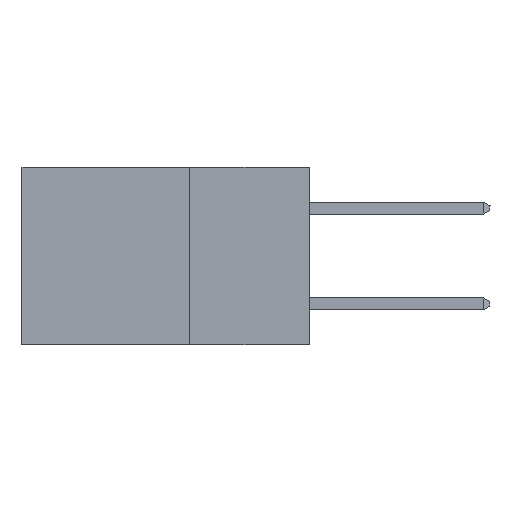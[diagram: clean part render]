
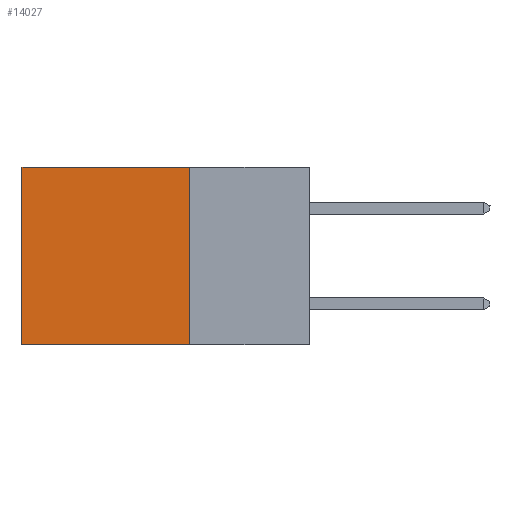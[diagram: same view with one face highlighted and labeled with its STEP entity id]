
A CAD part, left-side view. The second image highlights one B-rep face of the part: STEP entity #14027.
In plain terms, the highlighted planar face has unit normal (-1, 0, 0).
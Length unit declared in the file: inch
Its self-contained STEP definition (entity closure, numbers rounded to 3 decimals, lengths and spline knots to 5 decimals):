
#1872 = DIRECTION ( 'NONE',  ( 0., 1., 0. ) ) ;
#2733 = DIRECTION ( 'NONE',  ( 0., 0., -1. ) ) ;
#2737 = LINE ( 'NONE', #13166, #22405 ) ;
#5017 = AXIS2_PLACEMENT_3D ( 'NONE', #7949, #16722, #25868 ) ;
#5042 = EDGE_CURVE ( 'NONE', #13042, #8518, #17000, .T. ) ;
#5381 = DIRECTION ( 'NONE',  ( 0., 1., 0. ) ) ;
#6493 = EDGE_CURVE ( 'NONE', #26547, #13929, #2737, .T. ) ;
#7454 = PLANE ( 'NONE',  #5017 ) ;
#7816 = EDGE_CURVE ( 'NONE', #26547, #13042, #15989, .T. ) ;
#7836 = DIRECTION ( 'NONE',  ( 0., 0., -1. ) ) ;
#7949 = CARTESIAN_POINT ( 'NONE',  ( 0.2875, 0.25, 0. ) ) ;
#8518 = VERTEX_POINT ( 'NONE', #31159 ) ;
#8764 = ORIENTED_EDGE ( 'NONE', *, *, #28070, .F. ) ;
#11246 = CARTESIAN_POINT ( 'NONE',  ( 0.2875, 0.25, 0. ) ) ;
#12551 = VECTOR ( 'NONE', #5381, 39.37008 ) ;
#13042 = VERTEX_POINT ( 'NONE', #29510 ) ;
#13166 = CARTESIAN_POINT ( 'NONE',  ( 0.2875, 0.25, 0. ) ) ;
#13929 = VERTEX_POINT ( 'NONE', #28037 ) ;
#14027 = ADVANCED_FACE ( 'NONE', ( #21763 ), #7454, .F. ) ;
#15383 = ORIENTED_EDGE ( 'NONE', *, *, #7816, .T. ) ;
#15989 = LINE ( 'NONE', #32851, #12551 ) ;
#16722 = DIRECTION ( 'NONE',  ( 1., 0., 0. ) ) ;
#17000 = LINE ( 'NONE', #24329, #27331 ) ;
#18820 = ORIENTED_EDGE ( 'NONE', *, *, #6493, .F. ) ;
#20356 = EDGE_LOOP ( 'NONE', ( #22489, #8764, #18820, #15383 ) ) ;
#21763 = FACE_OUTER_BOUND ( 'NONE', #20356, .T. ) ;
#22405 = VECTOR ( 'NONE', #7836, 39.37008 ) ;
#22489 = ORIENTED_EDGE ( 'NONE', *, *, #5042, .T. ) ;
#24329 = CARTESIAN_POINT ( 'NONE',  ( 0.2875, 0.6, 0. ) ) ;
#25868 = DIRECTION ( 'NONE',  ( 0., 0., -1. ) ) ;
#26275 = CARTESIAN_POINT ( 'NONE',  ( 0.2875, 0.25, -0.37 ) ) ;
#26547 = VERTEX_POINT ( 'NONE', #11246 ) ;
#27109 = LINE ( 'NONE', #26275, #27969 ) ;
#27331 = VECTOR ( 'NONE', #2733, 39.37008 ) ;
#27969 = VECTOR ( 'NONE', #1872, 39.37008 ) ;
#28037 = CARTESIAN_POINT ( 'NONE',  ( 0.2875, 0.25, -0.37 ) ) ;
#28070 = EDGE_CURVE ( 'NONE', #13929, #8518, #27109, .T. ) ;
#29510 = CARTESIAN_POINT ( 'NONE',  ( 0.2875, 0.6, 0. ) ) ;
#31159 = CARTESIAN_POINT ( 'NONE',  ( 0.2875, 0.6, -0.37 ) ) ;
#32851 = CARTESIAN_POINT ( 'NONE',  ( 0.2875, 0.25, 0. ) ) ;
